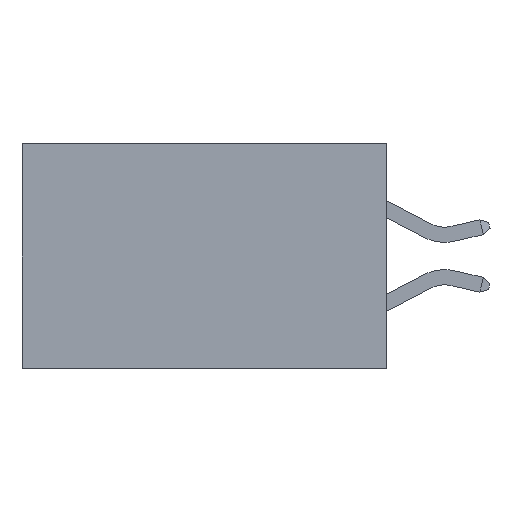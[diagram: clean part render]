
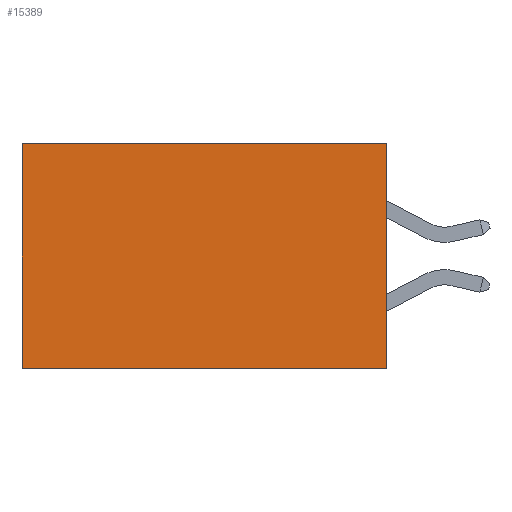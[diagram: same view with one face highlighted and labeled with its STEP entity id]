
A CAD part, left-side view. The second image highlights one B-rep face of the part: STEP entity #15389.
In plain terms, the highlighted planar face has unit normal (-1, 0, 0).
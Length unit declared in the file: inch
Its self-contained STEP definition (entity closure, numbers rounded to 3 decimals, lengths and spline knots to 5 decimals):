
#1365 = EDGE_CURVE ( 'NONE', #15442, #17927, #10926, .T. ) ;
#1634 = CARTESIAN_POINT ( 'NONE',  ( 0.2615, 0., -0.37 ) ) ;
#1847 = CARTESIAN_POINT ( 'NONE',  ( 0.2615, 0.6, -0.37 ) ) ;
#2097 = ORIENTED_EDGE ( 'NONE', *, *, #1365, .F. ) ;
#2269 = CARTESIAN_POINT ( 'NONE',  ( 0.2615, 0., -0.37 ) ) ;
#2769 = AXIS2_PLACEMENT_3D ( 'NONE', #2269, #4904, #17151 ) ;
#3198 = CARTESIAN_POINT ( 'NONE',  ( 0.2615, 0.6, -0.37 ) ) ;
#3706 = CARTESIAN_POINT ( 'NONE',  ( 0.2615, 0., -0.37 ) ) ;
#4037 = EDGE_CURVE ( 'NONE', #15442, #13877, #11282, .T. ) ;
#4246 = CARTESIAN_POINT ( 'NONE',  ( 0.2615, 0., -0.37 ) ) ;
#4389 = VECTOR ( 'NONE', #10722, 39.37008 ) ;
#4904 = DIRECTION ( 'NONE',  ( 1., 0., 0. ) ) ;
#5146 = VECTOR ( 'NONE', #14996, 39.37008 ) ;
#7362 = ORIENTED_EDGE ( 'NONE', *, *, #4037, .T. ) ;
#8009 = ORIENTED_EDGE ( 'NONE', *, *, #20247, .T. ) ;
#9153 = CARTESIAN_POINT ( 'NONE',  ( 0.2615, 0., 0. ) ) ;
#9665 = LINE ( 'NONE', #3198, #13590 ) ;
#9777 = DIRECTION ( 'NONE',  ( 0., 0., -1. ) ) ;
#10722 = DIRECTION ( 'NONE',  ( 0., 0., -1. ) ) ;
#10926 = LINE ( 'NONE', #4246, #4389 ) ;
#10957 = DIRECTION ( 'NONE',  ( 0., 1., 0. ) ) ;
#11282 = LINE ( 'NONE', #21015, #13765 ) ;
#11846 = EDGE_CURVE ( 'NONE', #17927, #13999, #16630, .T. ) ;
#12089 = PLANE ( 'NONE',  #2769 ) ;
#12442 = ORIENTED_EDGE ( 'NONE', *, *, #11846, .F. ) ;
#13590 = VECTOR ( 'NONE', #9777, 39.37008 ) ;
#13765 = VECTOR ( 'NONE', #10957, 39.37008 ) ;
#13877 = VERTEX_POINT ( 'NONE', #17792 ) ;
#13999 = VERTEX_POINT ( 'NONE', #1847 ) ;
#14592 = EDGE_LOOP ( 'NONE', ( #8009, #12442, #2097, #7362 ) ) ;
#14996 = DIRECTION ( 'NONE',  ( 0., 1., 0. ) ) ;
#15389 = ADVANCED_FACE ( 'NONE', ( #17052 ), #12089, .F. ) ;
#15442 = VERTEX_POINT ( 'NONE', #9153 ) ;
#16630 = LINE ( 'NONE', #1634, #5146 ) ;
#17052 = FACE_OUTER_BOUND ( 'NONE', #14592, .T. ) ;
#17151 = DIRECTION ( 'NONE',  ( 0., 0., -1. ) ) ;
#17792 = CARTESIAN_POINT ( 'NONE',  ( 0.2615, 0.6, 0. ) ) ;
#17927 = VERTEX_POINT ( 'NONE', #3706 ) ;
#20247 = EDGE_CURVE ( 'NONE', #13877, #13999, #9665, .T. ) ;
#21015 = CARTESIAN_POINT ( 'NONE',  ( 0.2615, 0., 0. ) ) ;
